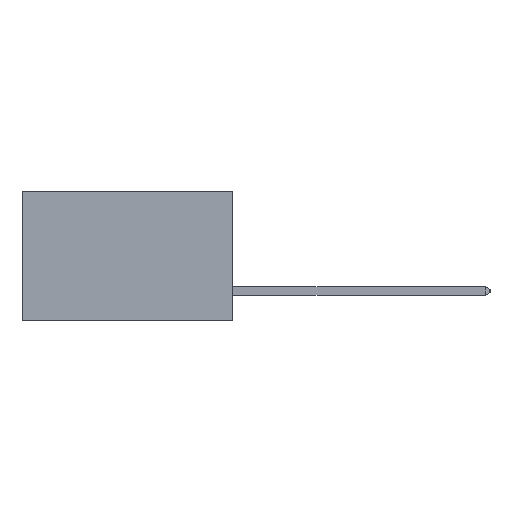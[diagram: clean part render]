
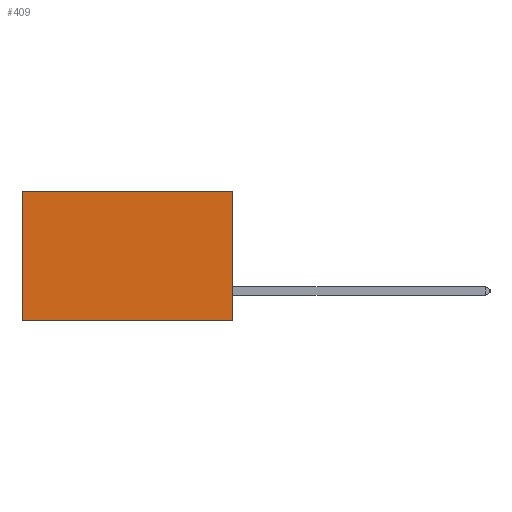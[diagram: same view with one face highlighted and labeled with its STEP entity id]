
A CAD part, left-side view. The second image highlights one B-rep face of the part: STEP entity #409.
In plain terms, the highlighted planar face has unit normal (-1, 0, 0).
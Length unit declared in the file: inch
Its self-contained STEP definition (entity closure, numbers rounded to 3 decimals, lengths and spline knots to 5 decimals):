
#409 = ADVANCED_FACE ( 'NONE', ( #25817 ), #20021, .F. ) ;
#1734 = LINE ( 'NONE', #36838, #14367 ) ;
#2586 = CARTESIAN_POINT ( 'NONE',  ( 0.2875, 0., -0.37 ) ) ;
#3301 = VECTOR ( 'NONE', #31870, 39.37008 ) ;
#4038 = CARTESIAN_POINT ( 'NONE',  ( 0.2875, 0.6, 0. ) ) ;
#5362 = ORIENTED_EDGE ( 'NONE', *, *, #23814, .T. ) ;
#5651 = EDGE_CURVE ( 'NONE', #10944, #10047, #20371, .T. ) ;
#6318 = VECTOR ( 'NONE', #33964, 39.37008 ) ;
#6326 = DIRECTION ( 'NONE',  ( 1., 0., 0. ) ) ;
#6714 = CARTESIAN_POINT ( 'NONE',  ( 0.2875, 0.6, -0.37 ) ) ;
#7226 = LINE ( 'NONE', #2586, #6318 ) ;
#9131 = CARTESIAN_POINT ( 'NONE',  ( 0.2875, 0., 0. ) ) ;
#10047 = VERTEX_POINT ( 'NONE', #17402 ) ;
#10944 = VERTEX_POINT ( 'NONE', #15738 ) ;
#11929 = EDGE_CURVE ( 'NONE', #10047, #14016, #7226, .T. ) ;
#12950 = VECTOR ( 'NONE', #30629, 39.37008 ) ;
#13296 = ORIENTED_EDGE ( 'NONE', *, *, #5651, .F. ) ;
#14016 = VERTEX_POINT ( 'NONE', #6714 ) ;
#14367 = VECTOR ( 'NONE', #17060, 39.37008 ) ;
#15738 = CARTESIAN_POINT ( 'NONE',  ( 0.2875, 0., 0. ) ) ;
#17060 = DIRECTION ( 'NONE',  ( 0., 0., -1. ) ) ;
#17402 = CARTESIAN_POINT ( 'NONE',  ( 0.2875, 0., -0.37 ) ) ;
#18209 = AXIS2_PLACEMENT_3D ( 'NONE', #18852, #6326, #29686 ) ;
#18511 = EDGE_LOOP ( 'NONE', ( #30097, #36671, #13296, #5362 ) ) ;
#18852 = CARTESIAN_POINT ( 'NONE',  ( 0.2875, 0., 0. ) ) ;
#20021 = PLANE ( 'NONE',  #18209 ) ;
#20371 = LINE ( 'NONE', #9131, #3301 ) ;
#20508 = LINE ( 'NONE', #36137, #12950 ) ;
#23152 = EDGE_CURVE ( 'NONE', #32175, #14016, #1734, .T. ) ;
#23814 = EDGE_CURVE ( 'NONE', #10944, #32175, #20508, .T. ) ;
#25817 = FACE_OUTER_BOUND ( 'NONE', #18511, .T. ) ;
#29686 = DIRECTION ( 'NONE',  ( 0., 0., -1. ) ) ;
#30097 = ORIENTED_EDGE ( 'NONE', *, *, #23152, .T. ) ;
#30629 = DIRECTION ( 'NONE',  ( 0., 1., 0. ) ) ;
#31870 = DIRECTION ( 'NONE',  ( 0., 0., -1. ) ) ;
#32175 = VERTEX_POINT ( 'NONE', #4038 ) ;
#33964 = DIRECTION ( 'NONE',  ( 0., 1., 0. ) ) ;
#36137 = CARTESIAN_POINT ( 'NONE',  ( 0.2875, 0., 0. ) ) ;
#36671 = ORIENTED_EDGE ( 'NONE', *, *, #11929, .F. ) ;
#36838 = CARTESIAN_POINT ( 'NONE',  ( 0.2875, 0.6, 0. ) ) ;
